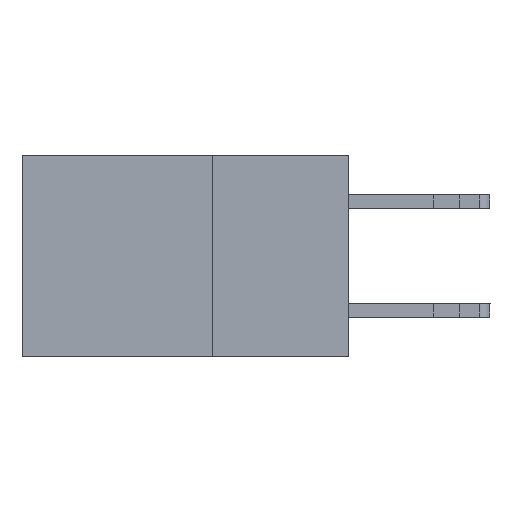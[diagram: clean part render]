
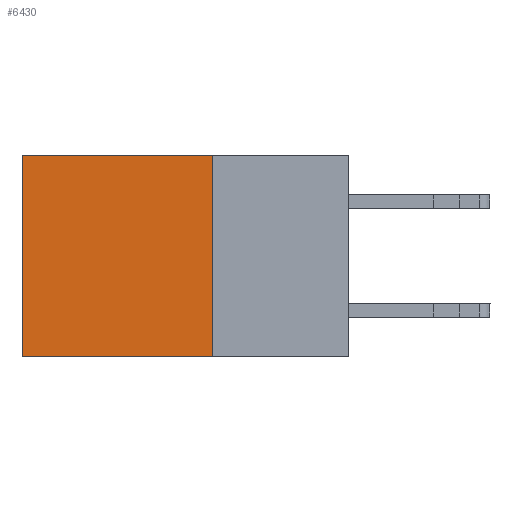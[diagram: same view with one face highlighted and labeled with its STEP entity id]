
A CAD part, left-side view. The second image highlights one B-rep face of the part: STEP entity #6430.
In plain terms, the highlighted planar face has unit normal (-1, 0, 0).
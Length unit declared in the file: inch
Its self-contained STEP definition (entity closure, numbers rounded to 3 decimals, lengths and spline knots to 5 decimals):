
#450 = ORIENTED_EDGE ( 'NONE', *, *, #8282, .F. ) ;
#470 = VECTOR ( 'NONE', #11349, 39.37008 ) ;
#548 = PLANE ( 'NONE',  #7369 ) ;
#1871 = EDGE_LOOP ( 'NONE', ( #3803, #4980, #450, #13091 ) ) ;
#1877 = EDGE_CURVE ( 'NONE', #10850, #5074, #4320, .T. ) ;
#1895 = DIRECTION ( 'NONE',  ( 1., 0., 0. ) ) ;
#3803 = ORIENTED_EDGE ( 'NONE', *, *, #1877, .T. ) ;
#3883 = CARTESIAN_POINT ( 'NONE',  ( 0.2615, 0.25, -0.37 ) ) ;
#4320 = LINE ( 'NONE', #10289, #6835 ) ;
#4791 = VERTEX_POINT ( 'NONE', #3883 ) ;
#4980 = ORIENTED_EDGE ( 'NONE', *, *, #10766, .F. ) ;
#5074 = VERTEX_POINT ( 'NONE', #7467 ) ;
#6030 = VECTOR ( 'NONE', #7965, 39.37008 ) ;
#6085 = EDGE_CURVE ( 'NONE', #8013, #10850, #11308, .T. ) ;
#6430 = ADVANCED_FACE ( 'NONE', ( #12497 ), #548, .F. ) ;
#6835 = VECTOR ( 'NONE', #11125, 39.37008 ) ;
#7369 = AXIS2_PLACEMENT_3D ( 'NONE', #8410, #1895, #9412 ) ;
#7467 = CARTESIAN_POINT ( 'NONE',  ( 0.2615, 0.6, -0.37 ) ) ;
#7965 = DIRECTION ( 'NONE',  ( 0., 0., -1. ) ) ;
#8013 = VERTEX_POINT ( 'NONE', #12489 ) ;
#8282 = EDGE_CURVE ( 'NONE', #8013, #4791, #13618, .T. ) ;
#8410 = CARTESIAN_POINT ( 'NONE',  ( 0.2615, 0.25, -0.37 ) ) ;
#9284 = VECTOR ( 'NONE', #12673, 39.37008 ) ;
#9412 = DIRECTION ( 'NONE',  ( 0., 0., -1. ) ) ;
#9979 = CARTESIAN_POINT ( 'NONE',  ( 0.2615, 0.25, -0.37 ) ) ;
#10289 = CARTESIAN_POINT ( 'NONE',  ( 0.2615, 0.6, -0.37 ) ) ;
#10766 = EDGE_CURVE ( 'NONE', #4791, #5074, #11692, .T. ) ;
#10850 = VERTEX_POINT ( 'NONE', #11434 ) ;
#11125 = DIRECTION ( 'NONE',  ( 0., 0., -1. ) ) ;
#11308 = LINE ( 'NONE', #13602, #9284 ) ;
#11349 = DIRECTION ( 'NONE',  ( 0., 1., 0. ) ) ;
#11434 = CARTESIAN_POINT ( 'NONE',  ( 0.2615, 0.6, 0. ) ) ;
#11692 = LINE ( 'NONE', #13266, #470 ) ;
#12489 = CARTESIAN_POINT ( 'NONE',  ( 0.2615, 0.25, 0. ) ) ;
#12497 = FACE_OUTER_BOUND ( 'NONE', #1871, .T. ) ;
#12673 = DIRECTION ( 'NONE',  ( 0., 1., 0. ) ) ;
#13091 = ORIENTED_EDGE ( 'NONE', *, *, #6085, .T. ) ;
#13266 = CARTESIAN_POINT ( 'NONE',  ( 0.2615, 0.25, -0.37 ) ) ;
#13602 = CARTESIAN_POINT ( 'NONE',  ( 0.2615, 0.25, 0. ) ) ;
#13618 = LINE ( 'NONE', #9979, #6030 ) ;
